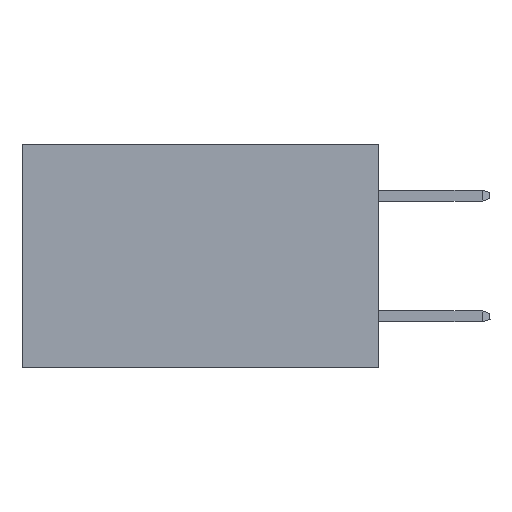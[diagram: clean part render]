
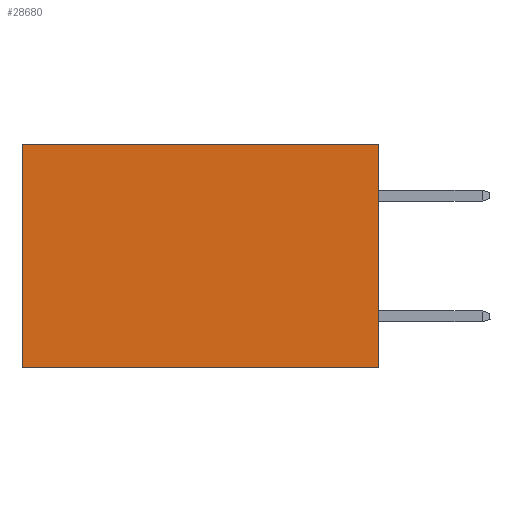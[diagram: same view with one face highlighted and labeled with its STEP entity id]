
A CAD part, left-side view. The second image highlights one B-rep face of the part: STEP entity #28680.
In plain terms, the highlighted planar face has unit normal (-1, 0, 0).
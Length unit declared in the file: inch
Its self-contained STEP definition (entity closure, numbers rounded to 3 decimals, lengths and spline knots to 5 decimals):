
#837 = ORIENTED_EDGE ( 'NONE', *, *, #20650, .F. ) ;
#876 = VERTEX_POINT ( 'NONE', #23210 ) ;
#1520 = CARTESIAN_POINT ( 'NONE',  ( 0.277, 0.59, -0.37 ) ) ;
#4932 = VECTOR ( 'NONE', #10617, 39.37008 ) ;
#5827 = VERTEX_POINT ( 'NONE', #22694 ) ;
#6076 = CARTESIAN_POINT ( 'NONE',  ( 0.277, 0.59, -0.37 ) ) ;
#6479 = CARTESIAN_POINT ( 'NONE',  ( 0.277, 0., 0. ) ) ;
#6843 = CARTESIAN_POINT ( 'NONE',  ( 0.277, 0., -0.37 ) ) ;
#7963 = ORIENTED_EDGE ( 'NONE', *, *, #16147, .F. ) ;
#8424 = DIRECTION ( 'NONE',  ( 0., 0., -1. ) ) ;
#9571 = LINE ( 'NONE', #29220, #16583 ) ;
#10559 = LINE ( 'NONE', #6076, #16094 ) ;
#10617 = DIRECTION ( 'NONE',  ( 0., 1., 0. ) ) ;
#10978 = EDGE_LOOP ( 'NONE', ( #12964, #837, #7963, #11228 ) ) ;
#11192 = LINE ( 'NONE', #19991, #4932 ) ;
#11228 = ORIENTED_EDGE ( 'NONE', *, *, #13779, .T. ) ;
#12928 = AXIS2_PLACEMENT_3D ( 'NONE', #13001, #29331, #15345 ) ;
#12964 = ORIENTED_EDGE ( 'NONE', *, *, #22403, .T. ) ;
#13001 = CARTESIAN_POINT ( 'NONE',  ( 0.277, 0., -0.37 ) ) ;
#13197 = FACE_OUTER_BOUND ( 'NONE', #10978, .T. ) ;
#13779 = EDGE_CURVE ( 'NONE', #25394, #5827, #11192, .T. ) ;
#15225 = DIRECTION ( 'NONE',  ( 0., 0., -1. ) ) ;
#15345 = DIRECTION ( 'NONE',  ( 0., 0., -1. ) ) ;
#16094 = VECTOR ( 'NONE', #8424, 39.37008 ) ;
#16147 = EDGE_CURVE ( 'NONE', #25394, #876, #9571, .T. ) ;
#16583 = VECTOR ( 'NONE', #15225, 39.37008 ) ;
#17610 = PLANE ( 'NONE',  #12928 ) ;
#19991 = CARTESIAN_POINT ( 'NONE',  ( 0.277, 0., 0. ) ) ;
#20650 = EDGE_CURVE ( 'NONE', #876, #28046, #21719, .T. ) ;
#20982 = VECTOR ( 'NONE', #25767, 39.37008 ) ;
#21719 = LINE ( 'NONE', #6843, #20982 ) ;
#22403 = EDGE_CURVE ( 'NONE', #5827, #28046, #10559, .T. ) ;
#22694 = CARTESIAN_POINT ( 'NONE',  ( 0.277, 0.59, 0. ) ) ;
#23210 = CARTESIAN_POINT ( 'NONE',  ( 0.277, 0., -0.37 ) ) ;
#25394 = VERTEX_POINT ( 'NONE', #6479 ) ;
#25767 = DIRECTION ( 'NONE',  ( 0., 1., 0. ) ) ;
#28046 = VERTEX_POINT ( 'NONE', #1520 ) ;
#28680 = ADVANCED_FACE ( 'NONE', ( #13197 ), #17610, .F. ) ;
#29220 = CARTESIAN_POINT ( 'NONE',  ( 0.277, 0., -0.37 ) ) ;
#29331 = DIRECTION ( 'NONE',  ( 1., 0., 0. ) ) ;
